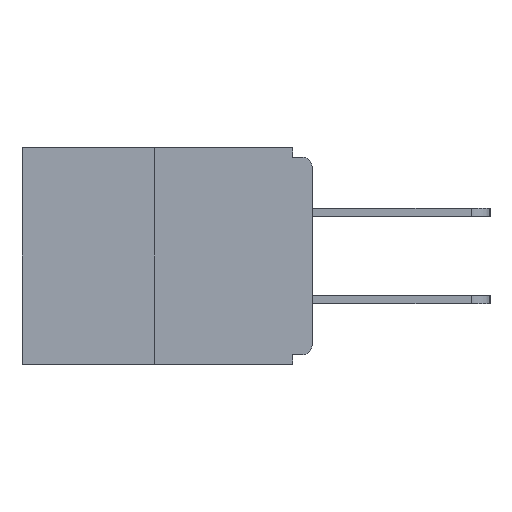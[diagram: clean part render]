
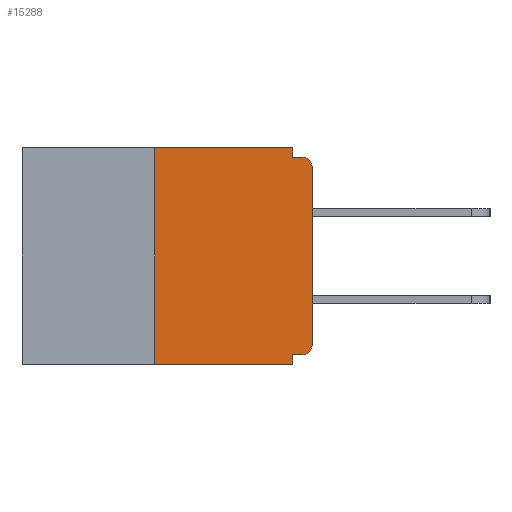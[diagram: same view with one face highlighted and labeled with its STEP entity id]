
A CAD part, left-side view. The second image highlights one B-rep face of the part: STEP entity #15288.
In plain terms, the highlighted planar face has unit normal (-1, 0, 0).
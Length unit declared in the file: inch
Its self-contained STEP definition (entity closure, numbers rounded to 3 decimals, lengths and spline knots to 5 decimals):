
#466 = EDGE_CURVE ( 'NONE', #7038, #13772, #1066, .T. ) ;
#944 = ORIENTED_EDGE ( 'NONE', *, *, #16152, .F. ) ;
#1066 = LINE ( 'NONE', #3840, #27082 ) ;
#1379 = EDGE_CURVE ( 'NONE', #19581, #7038, #21154, .T. ) ;
#1431 = DIRECTION ( 'NONE',  ( 0., 0., 1. ) ) ;
#1434 = DIRECTION ( 'NONE',  ( 0., -1., 0. ) ) ;
#1630 = ORIENTED_EDGE ( 'NONE', *, *, #12879, .F. ) ;
#1859 = ORIENTED_EDGE ( 'NONE', *, *, #10258, .T. ) ;
#2303 = DIRECTION ( 'NONE',  ( 0., 0., -1. ) ) ;
#2783 = LINE ( 'NONE', #18153, #14695 ) ;
#2810 = CARTESIAN_POINT ( 'NONE',  ( 0., 0.031, 0. ) ) ;
#2897 = CARTESIAN_POINT ( 'NONE',  ( 0., 0., -0.03 ) ) ;
#3060 = CARTESIAN_POINT ( 'NONE',  ( 0., 0.031, 0. ) ) ;
#3407 = CARTESIAN_POINT ( 'NONE',  ( 0., 0.46, 0. ) ) ;
#3496 = VERTEX_POINT ( 'NONE', #22095 ) ;
#3613 = VERTEX_POINT ( 'NONE', #20542 ) ;
#3701 = DIRECTION ( 'NONE',  ( 1., 0., 0. ) ) ;
#3840 = CARTESIAN_POINT ( 'NONE',  ( 0., 0.46, 0. ) ) ;
#3870 = DIRECTION ( 'NONE',  ( 0., 1., 0. ) ) ;
#4272 = ORIENTED_EDGE ( 'NONE', *, *, #20926, .F. ) ;
#4444 = VERTEX_POINT ( 'NONE', #2897 ) ;
#4929 = VERTEX_POINT ( 'NONE', #17847 ) ;
#5246 = DIRECTION ( 'NONE',  ( 0., 0., -1. ) ) ;
#5301 = FACE_OUTER_BOUND ( 'NONE', #5597, .T. ) ;
#5597 = EDGE_LOOP ( 'NONE', ( #19069, #19482, #18835, #1630, #4272, #9880, #1859, #26055, #944, #13993 ) ) ;
#5656 = CARTESIAN_POINT ( 'NONE',  ( 0., 0.46, -0.343 ) ) ;
#6852 = CIRCLE ( 'NONE', #7071, 0.015 ) ;
#7038 = VERTEX_POINT ( 'NONE', #24764 ) ;
#7071 = AXIS2_PLACEMENT_3D ( 'NONE', #13381, #21741, #26152 ) ;
#7092 = CARTESIAN_POINT ( 'NONE',  ( 0., 0.031, -0.015 ) ) ;
#7451 = CARTESIAN_POINT ( 'NONE',  ( 0., 0.25, 0. ) ) ;
#8558 = DIRECTION ( 'NONE',  ( 0., -1., 0. ) ) ;
#9880 = ORIENTED_EDGE ( 'NONE', *, *, #16365, .T. ) ;
#10258 = EDGE_CURVE ( 'NONE', #4929, #4444, #24939, .T. ) ;
#10807 = AXIS2_PLACEMENT_3D ( 'NONE', #26219, #23111, #18698 ) ;
#12787 = CARTESIAN_POINT ( 'NONE',  ( 0., 0., -0.328 ) ) ;
#12879 = EDGE_CURVE ( 'NONE', #3496, #22365, #2783, .T. ) ;
#13381 = CARTESIAN_POINT ( 'NONE',  ( 0., 0.015, -0.313 ) ) ;
#13772 = VERTEX_POINT ( 'NONE', #2810 ) ;
#13993 = ORIENTED_EDGE ( 'NONE', *, *, #18774, .F. ) ;
#14209 = PLANE ( 'NONE',  #22431 ) ;
#14695 = VECTOR ( 'NONE', #16346, 39.37008 ) ;
#15288 = ADVANCED_FACE ( 'NONE', ( #5301 ), #14209, .F. ) ;
#15305 = LINE ( 'NONE', #12787, #24144 ) ;
#15768 = VERTEX_POINT ( 'NONE', #7092 ) ;
#16012 = CARTESIAN_POINT ( 'NONE',  ( 0., 0.25, -0.343 ) ) ;
#16061 = LINE ( 'NONE', #3060, #21008 ) ;
#16151 = LINE ( 'NONE', #23049, #19735 ) ;
#16152 = EDGE_CURVE ( 'NONE', #15768, #3613, #16151, .T. ) ;
#16195 = CARTESIAN_POINT ( 'NONE',  ( 0., 0.015, -0.328 ) ) ;
#16346 = DIRECTION ( 'NONE',  ( 0., 0., -1. ) ) ;
#16365 = EDGE_CURVE ( 'NONE', #20154, #4929, #6852, .T. ) ;
#16471 = DIRECTION ( 'NONE',  ( 0., -1., 0. ) ) ;
#17685 = LINE ( 'NONE', #5656, #22656 ) ;
#17698 = VECTOR ( 'NONE', #20192, 39.37008 ) ;
#17847 = CARTESIAN_POINT ( 'NONE',  ( 0., 0., -0.313 ) ) ;
#18153 = CARTESIAN_POINT ( 'NONE',  ( 0., 0.031, -0.343 ) ) ;
#18698 = DIRECTION ( 'NONE',  ( 0., 0., -1. ) ) ;
#18774 = EDGE_CURVE ( 'NONE', #13772, #15768, #16061, .T. ) ;
#18835 = ORIENTED_EDGE ( 'NONE', *, *, #24042, .T. ) ;
#19069 = ORIENTED_EDGE ( 'NONE', *, *, #466, .F. ) ;
#19482 = ORIENTED_EDGE ( 'NONE', *, *, #1379, .F. ) ;
#19581 = VERTEX_POINT ( 'NONE', #16012 ) ;
#19735 = VECTOR ( 'NONE', #8558, 39.37008 ) ;
#20129 = CIRCLE ( 'NONE', #10807, 0.015 ) ;
#20154 = VERTEX_POINT ( 'NONE', #16195 ) ;
#20192 = DIRECTION ( 'NONE',  ( 0., 0., 1. ) ) ;
#20542 = CARTESIAN_POINT ( 'NONE',  ( 0., 0.015, -0.015 ) ) ;
#20926 = EDGE_CURVE ( 'NONE', #20154, #3496, #15305, .T. ) ;
#21008 = VECTOR ( 'NONE', #5246, 39.37008 ) ;
#21154 = LINE ( 'NONE', #7451, #21802 ) ;
#21741 = DIRECTION ( 'NONE',  ( -1., 0., 0. ) ) ;
#21802 = VECTOR ( 'NONE', #1431, 39.37008 ) ;
#22095 = CARTESIAN_POINT ( 'NONE',  ( 0., 0.031, -0.328 ) ) ;
#22179 = EDGE_CURVE ( 'NONE', #4444, #3613, #20129, .T. ) ;
#22226 = CARTESIAN_POINT ( 'NONE',  ( 0., 0., 0. ) ) ;
#22365 = VERTEX_POINT ( 'NONE', #26042 ) ;
#22431 = AXIS2_PLACEMENT_3D ( 'NONE', #3407, #3701, #2303 ) ;
#22656 = VECTOR ( 'NONE', #16471, 39.37008 ) ;
#23049 = CARTESIAN_POINT ( 'NONE',  ( 0., 0., -0.015 ) ) ;
#23111 = DIRECTION ( 'NONE',  ( -1., 0., 0. ) ) ;
#24042 = EDGE_CURVE ( 'NONE', #19581, #22365, #17685, .T. ) ;
#24144 = VECTOR ( 'NONE', #3870, 39.37008 ) ;
#24764 = CARTESIAN_POINT ( 'NONE',  ( 0., 0.25, 0. ) ) ;
#24939 = LINE ( 'NONE', #22226, #17698 ) ;
#26042 = CARTESIAN_POINT ( 'NONE',  ( 0., 0.031, -0.343 ) ) ;
#26055 = ORIENTED_EDGE ( 'NONE', *, *, #22179, .T. ) ;
#26152 = DIRECTION ( 'NONE',  ( 0., 0., -1. ) ) ;
#26219 = CARTESIAN_POINT ( 'NONE',  ( 0., 0.015, -0.03 ) ) ;
#27082 = VECTOR ( 'NONE', #1434, 39.37008 ) ;
